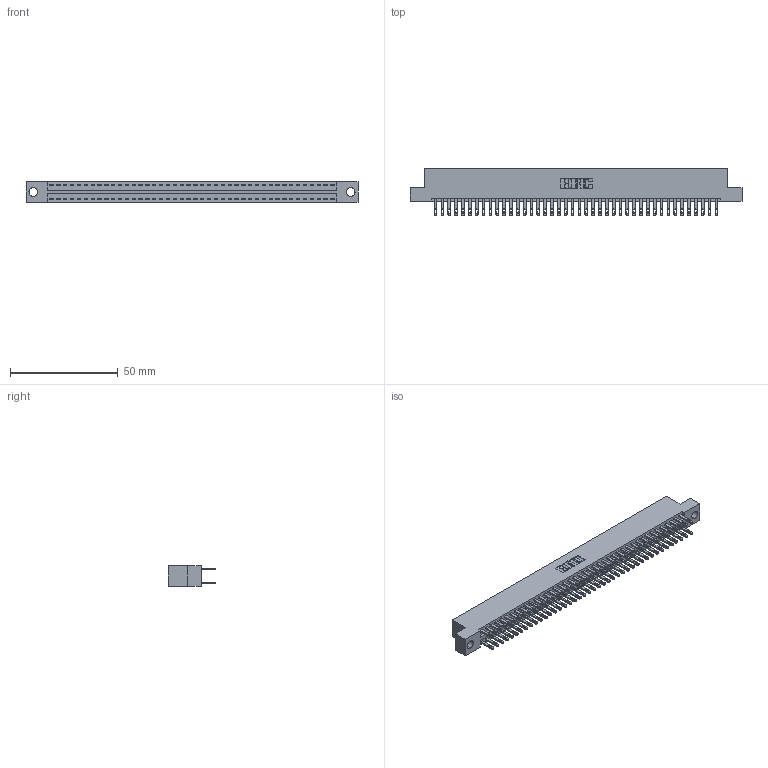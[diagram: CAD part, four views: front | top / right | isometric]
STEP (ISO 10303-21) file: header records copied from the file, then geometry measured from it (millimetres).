
FILE_DESCRIPTION (( 'STEP AP203' ), '1' );
FILE_NAME ('346-084-500-204.STEP', '2022-05-25T19:06:11', ( '' ), ( '' ), 'SwSTEP 2.0', 'SolidWorks 2020', '' );
FILE_SCHEMA (( 'CONFIG_CONTROL_DESIGN' ));
Length unit declared in the file: inch
Products named in the file (3): 346 Part_Flush Mounting Lugs - 0.156 Dia-TH; 346-084-500-204; 345-292-001_345-293-100
Assembly tree (85 placements, depth 2):
  346-084-500-204
    346 Part_Flush Mounting Lugs - 0.156 Dia-TH
    345-292-001_345-293-100  x84
Bounding box: 153.92 x 21.84 x 9.4 mm (x, y, z)
Volume: 15160.2 mm3; surface area: 21565.8 mm2
Topology: 85 solids, 85 shells, 4168 faces, 12713 edges, 8474 vertices
Faces by surface type: plane 2526, cylinder 1642
Entity records: 27759 total; most frequent: CARTESIAN_POINT 4578, ORIENTED_EDGE 4510, DIRECTION 4087, EDGE_CURVE 2255, VECTOR 1951, LINE 1951, VERTEX_POINT 1502, AXIS2_PLACEMENT_3D 1068
